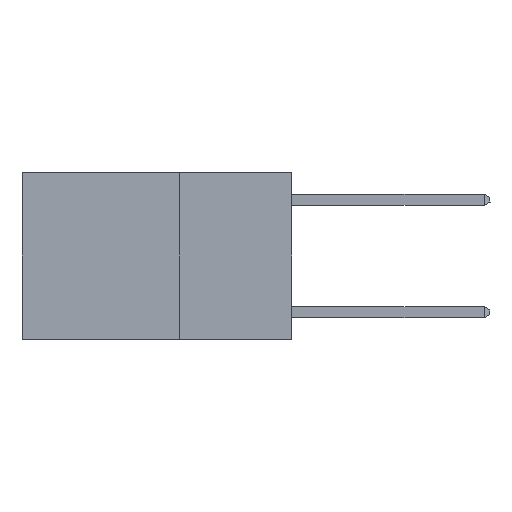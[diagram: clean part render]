
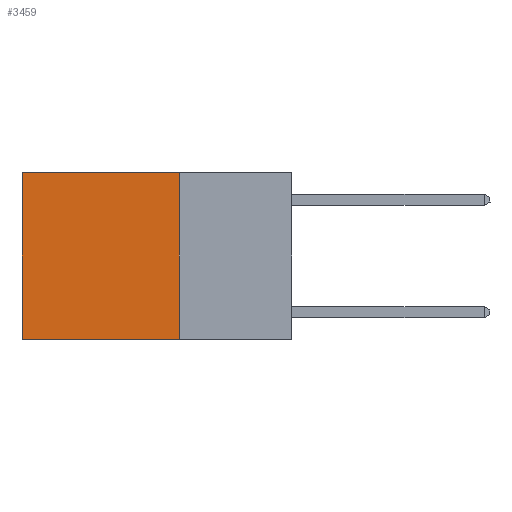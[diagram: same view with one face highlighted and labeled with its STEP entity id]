
A CAD part, left-side view. The second image highlights one B-rep face of the part: STEP entity #3459.
In plain terms, the highlighted planar face has unit normal (-1, 0, 0).
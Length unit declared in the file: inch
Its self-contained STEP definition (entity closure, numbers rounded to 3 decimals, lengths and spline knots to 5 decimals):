
#172 = ORIENTED_EDGE ( 'NONE', *, *, #7579, .F. ) ;
#465 = CARTESIAN_POINT ( 'NONE',  ( 0.2625, 0.6, 0. ) ) ;
#655 = PLANE ( 'NONE',  #9683 ) ;
#682 = ORIENTED_EDGE ( 'NONE', *, *, #3824, .T. ) ;
#869 = LINE ( 'NONE', #7480, #7983 ) ;
#1159 = VERTEX_POINT ( 'NONE', #8975 ) ;
#3161 = VERTEX_POINT ( 'NONE', #7684 ) ;
#3232 = CARTESIAN_POINT ( 'NONE',  ( 0.2625, 0.25, -0.37 ) ) ;
#3459 = ADVANCED_FACE ( 'NONE', ( #9206 ), #655, .F. ) ;
#3715 = CARTESIAN_POINT ( 'NONE',  ( 0.2625, 0.6, 0. ) ) ;
#3824 = EDGE_CURVE ( 'NONE', #3161, #6938, #10272, .T. ) ;
#4043 = CARTESIAN_POINT ( 'NONE',  ( 0.2625, 0.25, 0. ) ) ;
#4988 = DIRECTION ( 'NONE',  ( 0., 0., -1. ) ) ;
#5379 = ORIENTED_EDGE ( 'NONE', *, *, #6228, .T. ) ;
#5399 = EDGE_CURVE ( 'NONE', #3161, #8018, #10619, .T. ) ;
#5402 = CARTESIAN_POINT ( 'NONE',  ( 0.2625, 0.25, 0. ) ) ;
#5923 = EDGE_LOOP ( 'NONE', ( #5379, #172, #6733, #682 ) ) ;
#6228 = EDGE_CURVE ( 'NONE', #6938, #1159, #7990, .T. ) ;
#6366 = DIRECTION ( 'NONE',  ( 0., 0., -1. ) ) ;
#6733 = ORIENTED_EDGE ( 'NONE', *, *, #5399, .F. ) ;
#6773 = DIRECTION ( 'NONE',  ( 0., 1., 0. ) ) ;
#6938 = VERTEX_POINT ( 'NONE', #465 ) ;
#7480 = CARTESIAN_POINT ( 'NONE',  ( 0.2625, 0.25, -0.37 ) ) ;
#7530 = VECTOR ( 'NONE', #10439, 39.37008 ) ;
#7579 = EDGE_CURVE ( 'NONE', #8018, #1159, #869, .T. ) ;
#7684 = CARTESIAN_POINT ( 'NONE',  ( 0.2625, 0.25, 0. ) ) ;
#7983 = VECTOR ( 'NONE', #6773, 39.37008 ) ;
#7990 = LINE ( 'NONE', #3715, #9277 ) ;
#8018 = VERTEX_POINT ( 'NONE', #3232 ) ;
#8178 = DIRECTION ( 'NONE',  ( 1., 0., 0. ) ) ;
#8272 = VECTOR ( 'NONE', #4988, 39.37008 ) ;
#8893 = CARTESIAN_POINT ( 'NONE',  ( 0.2625, 0.25, 0. ) ) ;
#8975 = CARTESIAN_POINT ( 'NONE',  ( 0.2625, 0.6, -0.37 ) ) ;
#8994 = DIRECTION ( 'NONE',  ( 0., 0., -1. ) ) ;
#9206 = FACE_OUTER_BOUND ( 'NONE', #5923, .T. ) ;
#9277 = VECTOR ( 'NONE', #6366, 39.37008 ) ;
#9683 = AXIS2_PLACEMENT_3D ( 'NONE', #8893, #8178, #8994 ) ;
#10272 = LINE ( 'NONE', #5402, #7530 ) ;
#10439 = DIRECTION ( 'NONE',  ( 0., 1., 0. ) ) ;
#10619 = LINE ( 'NONE', #4043, #8272 ) ;
